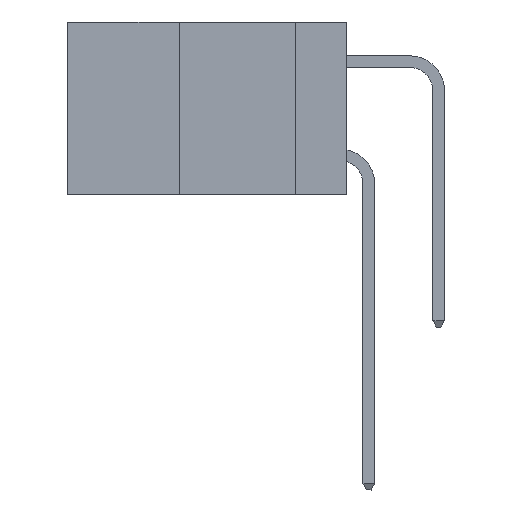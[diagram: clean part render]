
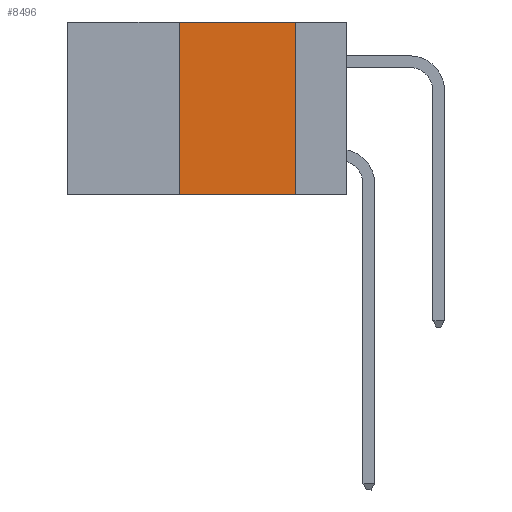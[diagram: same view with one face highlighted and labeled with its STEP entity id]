
A CAD part, left-side view. The second image highlights one B-rep face of the part: STEP entity #8496.
In plain terms, the highlighted planar face has unit normal (-1, 0, 0).
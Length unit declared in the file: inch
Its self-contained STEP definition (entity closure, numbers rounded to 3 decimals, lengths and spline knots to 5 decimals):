
#331 = VECTOR ( 'NONE', #2681, 39.37008 ) ;
#695 = LINE ( 'NONE', #16200, #14403 ) ;
#1853 = VERTEX_POINT ( 'NONE', #1985 ) ;
#1985 = CARTESIAN_POINT ( 'NONE',  ( 0., 0.36, 0. ) ) ;
#2681 = DIRECTION ( 'NONE',  ( 0., -1., 0. ) ) ;
#3007 = VECTOR ( 'NONE', #8686, 39.37008 ) ;
#3041 = CARTESIAN_POINT ( 'NONE',  ( 0., 0.11, 0. ) ) ;
#3657 = EDGE_CURVE ( 'NONE', #1853, #17096, #11598, .T. ) ;
#4894 = EDGE_CURVE ( 'NONE', #10057, #13407, #7027, .T. ) ;
#5263 = ORIENTED_EDGE ( 'NONE', *, *, #4894, .T. ) ;
#5856 = CARTESIAN_POINT ( 'NONE',  ( 0., 0.11, 0. ) ) ;
#6416 = DIRECTION ( 'NONE',  ( 0., 0., 1. ) ) ;
#7027 = LINE ( 'NONE', #9283, #331 ) ;
#7465 = EDGE_LOOP ( 'NONE', ( #10846, #9963, #9981, #5263 ) ) ;
#8496 = ADVANCED_FACE ( 'NONE', ( #15053 ), #12373, .F. ) ;
#8686 = DIRECTION ( 'NONE',  ( 0., 0., -1. ) ) ;
#8740 = EDGE_CURVE ( 'NONE', #17096, #13407, #17552, .T. ) ;
#9283 = CARTESIAN_POINT ( 'NONE',  ( 0., 0.6, -0.37 ) ) ;
#9963 = ORIENTED_EDGE ( 'NONE', *, *, #3657, .F. ) ;
#9981 = ORIENTED_EDGE ( 'NONE', *, *, #12580, .F. ) ;
#10057 = VERTEX_POINT ( 'NONE', #11102 ) ;
#10578 = AXIS2_PLACEMENT_3D ( 'NONE', #10822, #15150, #16436 ) ;
#10822 = CARTESIAN_POINT ( 'NONE',  ( 0., 0.6, 0. ) ) ;
#10846 = ORIENTED_EDGE ( 'NONE', *, *, #8740, .F. ) ;
#11082 = VECTOR ( 'NONE', #13235, 39.37008 ) ;
#11102 = CARTESIAN_POINT ( 'NONE',  ( 0., 0.36, -0.37 ) ) ;
#11598 = LINE ( 'NONE', #17324, #11082 ) ;
#12373 = PLANE ( 'NONE',  #10578 ) ;
#12580 = EDGE_CURVE ( 'NONE', #10057, #1853, #695, .T. ) ;
#13235 = DIRECTION ( 'NONE',  ( 0., -1., 0. ) ) ;
#13407 = VERTEX_POINT ( 'NONE', #16131 ) ;
#14403 = VECTOR ( 'NONE', #6416, 39.37008 ) ;
#15053 = FACE_OUTER_BOUND ( 'NONE', #7465, .T. ) ;
#15150 = DIRECTION ( 'NONE',  ( 1., 0., 0. ) ) ;
#16131 = CARTESIAN_POINT ( 'NONE',  ( 0., 0.11, -0.37 ) ) ;
#16200 = CARTESIAN_POINT ( 'NONE',  ( 0., 0.36, 0. ) ) ;
#16436 = DIRECTION ( 'NONE',  ( 0., 0., -1. ) ) ;
#17096 = VERTEX_POINT ( 'NONE', #5856 ) ;
#17324 = CARTESIAN_POINT ( 'NONE',  ( 0., 0.6, 0. ) ) ;
#17552 = LINE ( 'NONE', #3041, #3007 ) ;
